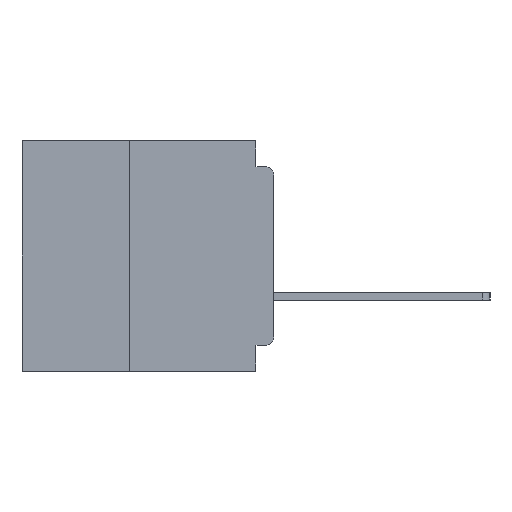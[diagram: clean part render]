
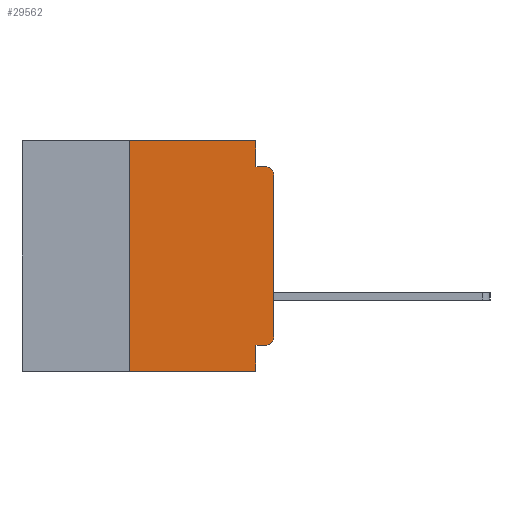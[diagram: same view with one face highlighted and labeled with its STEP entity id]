
A CAD part, left-side view. The second image highlights one B-rep face of the part: STEP entity #29562.
In plain terms, the highlighted planar face has unit normal (-1, 0, 0).
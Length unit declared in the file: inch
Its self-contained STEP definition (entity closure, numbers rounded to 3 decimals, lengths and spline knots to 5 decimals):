
#995 = DIRECTION ( 'NONE',  ( 0., -1., 0. ) ) ;
#1533 = DIRECTION ( 'NONE',  ( -1., 0., 0. ) ) ;
#1990 = DIRECTION ( 'NONE',  ( 0., 0., -1. ) ) ;
#2284 = AXIS2_PLACEMENT_3D ( 'NONE', #17825, #1533, #20520 ) ;
#2544 = LINE ( 'NONE', #20389, #21590 ) ;
#2692 = CARTESIAN_POINT ( 'NONE',  ( 0., 0.25, 0. ) ) ;
#3476 = LINE ( 'NONE', #29468, #17882 ) ;
#3904 = DIRECTION ( 'NONE',  ( 0., -1., 0. ) ) ;
#4191 = LINE ( 'NONE', #22798, #10585 ) ;
#4738 = VECTOR ( 'NONE', #23248, 39.37008 ) ;
#5838 = DIRECTION ( 'NONE',  ( 0., 0., 1. ) ) ;
#6071 = EDGE_LOOP ( 'NONE', ( #15223, #11975, #14777, #34122, #32408, #6898, #20715, #17034, #26647, #18298 ) ) ;
#6183 = VERTEX_POINT ( 'NONE', #24003 ) ;
#6225 = EDGE_CURVE ( 'NONE', #14767, #14920, #3476, .T. ) ;
#6598 = VERTEX_POINT ( 'NONE', #25728 ) ;
#6839 = PLANE ( 'NONE',  #15013 ) ;
#6898 = ORIENTED_EDGE ( 'NONE', *, *, #33093, .F. ) ;
#6977 = DIRECTION ( 'NONE',  ( 0., 0., -1. ) ) ;
#7443 = VECTOR ( 'NONE', #5838, 39.37008 ) ;
#7907 = DIRECTION ( 'NONE',  ( 0., 1., 0. ) ) ;
#7980 = EDGE_CURVE ( 'NONE', #10654, #6183, #9380, .T. ) ;
#8020 = DIRECTION ( 'NONE',  ( 0., 0., -1. ) ) ;
#9012 = CARTESIAN_POINT ( 'NONE',  ( 0., 0.031, 0. ) ) ;
#9185 = CIRCLE ( 'NONE', #2284, 0.015 ) ;
#9380 = LINE ( 'NONE', #18762, #15715 ) ;
#9873 = VECTOR ( 'NONE', #34294, 39.37008 ) ;
#10585 = VECTOR ( 'NONE', #3904, 39.37008 ) ;
#10654 = VERTEX_POINT ( 'NONE', #9012 ) ;
#11613 = VERTEX_POINT ( 'NONE', #22951 ) ;
#11975 = ORIENTED_EDGE ( 'NONE', *, *, #29712, .T. ) ;
#12160 = EDGE_CURVE ( 'NONE', #6183, #11613, #12284, .T. ) ;
#12201 = EDGE_CURVE ( 'NONE', #12555, #21284, #4191, .T. ) ;
#12284 = LINE ( 'NONE', #33197, #33534 ) ;
#12286 = DIRECTION ( 'NONE',  ( 0., 0., -1. ) ) ;
#12555 = VERTEX_POINT ( 'NONE', #32134 ) ;
#13040 = CARTESIAN_POINT ( 'NONE',  ( 0., 0., 0. ) ) ;
#14401 = CARTESIAN_POINT ( 'NONE',  ( 0., 0., -0.34 ) ) ;
#14767 = VERTEX_POINT ( 'NONE', #25666 ) ;
#14777 = ORIENTED_EDGE ( 'NONE', *, *, #12160, .F. ) ;
#14920 = VERTEX_POINT ( 'NONE', #18416 ) ;
#15013 = AXIS2_PLACEMENT_3D ( 'NONE', #25645, #28326, #12286 ) ;
#15223 = ORIENTED_EDGE ( 'NONE', *, *, #29113, .T. ) ;
#15715 = VECTOR ( 'NONE', #8020, 39.37008 ) ;
#15753 = VERTEX_POINT ( 'NONE', #14401 ) ;
#17034 = ORIENTED_EDGE ( 'NONE', *, *, #23531, .F. ) ;
#17825 = CARTESIAN_POINT ( 'NONE',  ( 0., 0.015, -0.34 ) ) ;
#17867 = CARTESIAN_POINT ( 'NONE',  ( 0., 0.437, 0. ) ) ;
#17869 = EDGE_CURVE ( 'NONE', #33001, #10654, #26236, .T. ) ;
#17882 = VECTOR ( 'NONE', #7907, 39.37008 ) ;
#18269 = DIRECTION ( 'NONE',  ( -1., 0., 0. ) ) ;
#18298 = ORIENTED_EDGE ( 'NONE', *, *, #22005, .T. ) ;
#18416 = CARTESIAN_POINT ( 'NONE',  ( 0., 0.031, -0.355 ) ) ;
#18762 = CARTESIAN_POINT ( 'NONE',  ( 0., 0.031, 0. ) ) ;
#20386 = AXIS2_PLACEMENT_3D ( 'NONE', #34146, #18269, #1990 ) ;
#20389 = CARTESIAN_POINT ( 'NONE',  ( 0., 0.031, -0.4 ) ) ;
#20520 = DIRECTION ( 'NONE',  ( 0., 0., -1. ) ) ;
#20715 = ORIENTED_EDGE ( 'NONE', *, *, #12201, .T. ) ;
#20771 = FACE_OUTER_BOUND ( 'NONE', #6071, .T. ) ;
#21284 = VERTEX_POINT ( 'NONE', #22793 ) ;
#21590 = VECTOR ( 'NONE', #6977, 39.37008 ) ;
#21749 = LINE ( 'NONE', #29999, #7443 ) ;
#22005 = EDGE_CURVE ( 'NONE', #14767, #15753, #9185, .T. ) ;
#22793 = CARTESIAN_POINT ( 'NONE',  ( 0., 0.031, -0.4 ) ) ;
#22798 = CARTESIAN_POINT ( 'NONE',  ( 0., 0.437, -0.4 ) ) ;
#22858 = CIRCLE ( 'NONE', #20386, 0.015 ) ;
#22951 = CARTESIAN_POINT ( 'NONE',  ( 0., 0.015, -0.045 ) ) ;
#23248 = DIRECTION ( 'NONE',  ( 0., -1., 0. ) ) ;
#23304 = LINE ( 'NONE', #13040, #9873 ) ;
#23531 = EDGE_CURVE ( 'NONE', #14920, #21284, #2544, .T. ) ;
#24003 = CARTESIAN_POINT ( 'NONE',  ( 0., 0.031, -0.045 ) ) ;
#25645 = CARTESIAN_POINT ( 'NONE',  ( 0., 0.437, 0. ) ) ;
#25666 = CARTESIAN_POINT ( 'NONE',  ( 0., 0.015, -0.355 ) ) ;
#25728 = CARTESIAN_POINT ( 'NONE',  ( 0., 0., -0.06 ) ) ;
#26236 = LINE ( 'NONE', #17867, #4738 ) ;
#26647 = ORIENTED_EDGE ( 'NONE', *, *, #6225, .F. ) ;
#28326 = DIRECTION ( 'NONE',  ( 1., 0., 0. ) ) ;
#29113 = EDGE_CURVE ( 'NONE', #15753, #6598, #23304, .T. ) ;
#29468 = CARTESIAN_POINT ( 'NONE',  ( 0., 0., -0.355 ) ) ;
#29562 = ADVANCED_FACE ( 'NONE', ( #20771 ), #6839, .F. ) ;
#29712 = EDGE_CURVE ( 'NONE', #6598, #11613, #22858, .T. ) ;
#29999 = CARTESIAN_POINT ( 'NONE',  ( 0., 0.25, -0.4 ) ) ;
#32134 = CARTESIAN_POINT ( 'NONE',  ( 0., 0.25, -0.4 ) ) ;
#32408 = ORIENTED_EDGE ( 'NONE', *, *, #17869, .F. ) ;
#33001 = VERTEX_POINT ( 'NONE', #2692 ) ;
#33093 = EDGE_CURVE ( 'NONE', #12555, #33001, #21749, .T. ) ;
#33197 = CARTESIAN_POINT ( 'NONE',  ( 0., 0., -0.045 ) ) ;
#33534 = VECTOR ( 'NONE', #995, 39.37008 ) ;
#34122 = ORIENTED_EDGE ( 'NONE', *, *, #7980, .F. ) ;
#34146 = CARTESIAN_POINT ( 'NONE',  ( 0., 0.015, -0.06 ) ) ;
#34294 = DIRECTION ( 'NONE',  ( 0., 0., 1. ) ) ;
